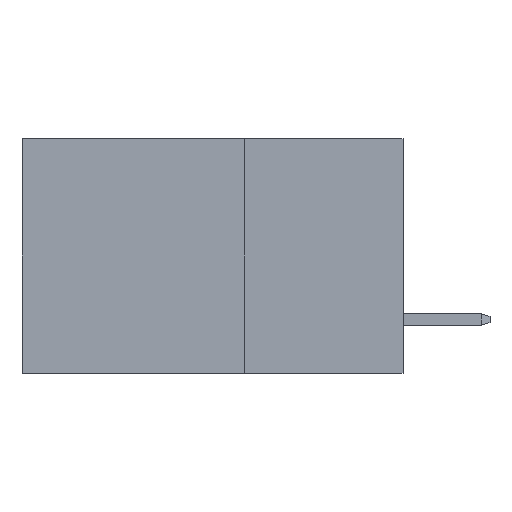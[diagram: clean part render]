
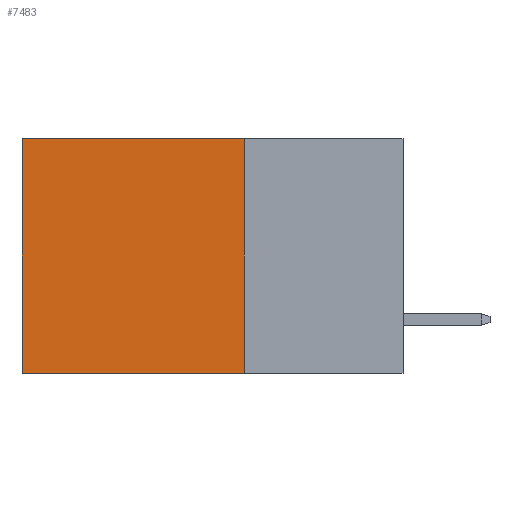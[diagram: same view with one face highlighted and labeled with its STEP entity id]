
A CAD part, left-side view. The second image highlights one B-rep face of the part: STEP entity #7483.
In plain terms, the highlighted planar face has unit normal (-1, 0, 0).
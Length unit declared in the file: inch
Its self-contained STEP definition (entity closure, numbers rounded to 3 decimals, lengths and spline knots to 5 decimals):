
#159 = VERTEX_POINT ( 'NONE', #1747 ) ;
#229 = VECTOR ( 'NONE', #8487, 39.37008 ) ;
#251 = EDGE_CURVE ( 'NONE', #159, #4360, #1035, .T. ) ;
#399 = EDGE_CURVE ( 'NONE', #6259, #159, #8523, .T. ) ;
#1035 = LINE ( 'NONE', #8902, #9978 ) ;
#1541 = CARTESIAN_POINT ( 'NONE',  ( 0.2875, 0.25, 0. ) ) ;
#1747 = CARTESIAN_POINT ( 'NONE',  ( 0.2875, 0.25, -0.37 ) ) ;
#2354 = FACE_OUTER_BOUND ( 'NONE', #8827, .T. ) ;
#3606 = EDGE_CURVE ( 'NONE', #6259, #4942, #4554, .T. ) ;
#3630 = VECTOR ( 'NONE', #6592, 39.37008 ) ;
#3673 = DIRECTION ( 'NONE',  ( 0., 0., -1. ) ) ;
#4145 = EDGE_CURVE ( 'NONE', #4942, #4360, #8156, .T. ) ;
#4360 = VERTEX_POINT ( 'NONE', #7837 ) ;
#4554 = LINE ( 'NONE', #6047, #229 ) ;
#4942 = VERTEX_POINT ( 'NONE', #6717 ) ;
#4992 = CARTESIAN_POINT ( 'NONE',  ( 0.2875, 0.25, 0. ) ) ;
#5475 = PLANE ( 'NONE',  #8167 ) ;
#5495 = ORIENTED_EDGE ( 'NONE', *, *, #251, .F. ) ;
#5837 = DIRECTION ( 'NONE',  ( 0., 1., 0. ) ) ;
#6039 = ORIENTED_EDGE ( 'NONE', *, *, #4145, .T. ) ;
#6047 = CARTESIAN_POINT ( 'NONE',  ( 0.2875, 0.25, 0. ) ) ;
#6173 = CARTESIAN_POINT ( 'NONE',  ( 0.2875, 0.25, 0. ) ) ;
#6184 = DIRECTION ( 'NONE',  ( 1., 0., 0. ) ) ;
#6259 = VERTEX_POINT ( 'NONE', #4992 ) ;
#6395 = VECTOR ( 'NONE', #3673, 39.37008 ) ;
#6592 = DIRECTION ( 'NONE',  ( 0., 0., -1. ) ) ;
#6717 = CARTESIAN_POINT ( 'NONE',  ( 0.2875, 0.6, 0. ) ) ;
#7351 = CARTESIAN_POINT ( 'NONE',  ( 0.2875, 0.6, 0. ) ) ;
#7483 = ADVANCED_FACE ( 'NONE', ( #2354 ), #5475, .F. ) ;
#7837 = CARTESIAN_POINT ( 'NONE',  ( 0.2875, 0.6, -0.37 ) ) ;
#7911 = DIRECTION ( 'NONE',  ( 0., 0., -1. ) ) ;
#8156 = LINE ( 'NONE', #7351, #3630 ) ;
#8167 = AXIS2_PLACEMENT_3D ( 'NONE', #1541, #6184, #7911 ) ;
#8307 = ORIENTED_EDGE ( 'NONE', *, *, #3606, .T. ) ;
#8487 = DIRECTION ( 'NONE',  ( 0., 1., 0. ) ) ;
#8523 = LINE ( 'NONE', #6173, #6395 ) ;
#8827 = EDGE_LOOP ( 'NONE', ( #6039, #5495, #9760, #8307 ) ) ;
#8902 = CARTESIAN_POINT ( 'NONE',  ( 0.2875, 0.25, -0.37 ) ) ;
#9760 = ORIENTED_EDGE ( 'NONE', *, *, #399, .F. ) ;
#9978 = VECTOR ( 'NONE', #5837, 39.37008 ) ;
